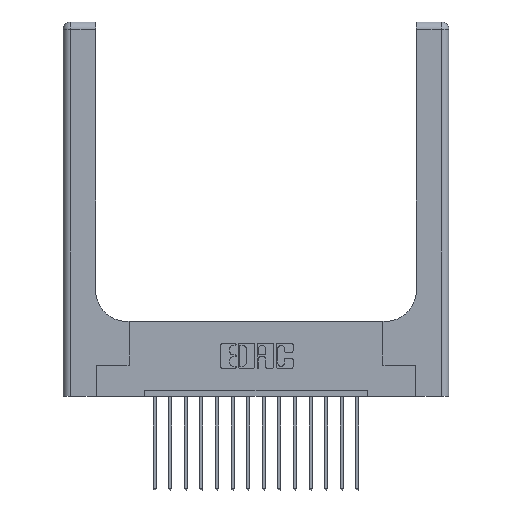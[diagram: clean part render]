
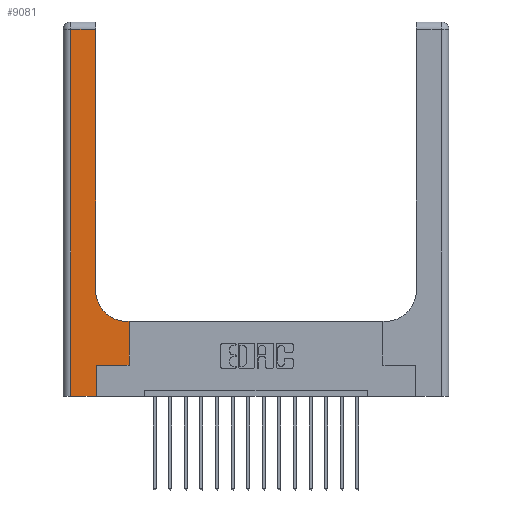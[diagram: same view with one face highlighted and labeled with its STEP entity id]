
A CAD part, top view. The second image highlights one B-rep face of the part: STEP entity #9081.
In plain terms, the highlighted planar face has unit normal (0, 0, 1).
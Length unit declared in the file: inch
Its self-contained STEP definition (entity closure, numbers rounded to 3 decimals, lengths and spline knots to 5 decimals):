
#2 = VECTOR ( 'NONE', #9991, 39.37008 ) ;
#161 = ORIENTED_EDGE ( 'NONE', *, *, #17061, .T. ) ;
#279 = EDGE_LOOP ( 'NONE', ( #14642, #14988, #15880, #3249, #939, #161, #603, #3914, #4945 ) ) ;
#603 = ORIENTED_EDGE ( 'NONE', *, *, #10340, .T. ) ;
#939 = ORIENTED_EDGE ( 'NONE', *, *, #5031, .T. ) ;
#1155 = CARTESIAN_POINT ( 'NONE',  ( 0.528, 0.25, 0.37 ) ) ;
#1302 = DIRECTION ( 'NONE',  ( 0., 1., 0. ) ) ;
#1533 = EDGE_CURVE ( 'NONE', #13329, #9422, #11969, .T. ) ;
#1597 = VECTOR ( 'NONE', #3873, 39.37008 ) ;
#1811 = DIRECTION ( 'NONE',  ( 0., 0., -1. ) ) ;
#2085 = CARTESIAN_POINT ( 'NONE',  ( 0.26, 2.94, 0.37 ) ) ;
#2169 = VECTOR ( 'NONE', #1302, 39.37008 ) ;
#2172 = CARTESIAN_POINT ( 'NONE',  ( 0.06, 2.94, 0.37 ) ) ;
#2354 = VERTEX_POINT ( 'NONE', #2085 ) ;
#2669 = DIRECTION ( 'NONE',  ( 0., 0., -1. ) ) ;
#2956 = LINE ( 'NONE', #17165, #17022 ) ;
#2967 = VERTEX_POINT ( 'NONE', #2172 ) ;
#2977 = CARTESIAN_POINT ( 'NONE',  ( 0., 0., 0.37 ) ) ;
#3102 = VERTEX_POINT ( 'NONE', #13186 ) ;
#3125 = PLANE ( 'NONE',  #13620 ) ;
#3194 = DIRECTION ( 'NONE',  ( 0., -1., 0. ) ) ;
#3249 = ORIENTED_EDGE ( 'NONE', *, *, #1533, .T. ) ;
#3291 = CARTESIAN_POINT ( 'NONE',  ( 0.06, 0., 0.37 ) ) ;
#3873 = DIRECTION ( 'NONE',  ( 0., 1., 0. ) ) ;
#3914 = ORIENTED_EDGE ( 'NONE', *, *, #6206, .T. ) ;
#3915 = CARTESIAN_POINT ( 'NONE',  ( 0.528, 0.25, 0.37 ) ) ;
#4129 = CARTESIAN_POINT ( 'NONE',  ( 0., 2.94, 0.37 ) ) ;
#4898 = DIRECTION ( 'NONE',  ( 1., 0., 0. ) ) ;
#4945 = ORIENTED_EDGE ( 'NONE', *, *, #11742, .T. ) ;
#4989 = VECTOR ( 'NONE', #12416, 39.37008 ) ;
#5031 = EDGE_CURVE ( 'NONE', #9422, #11047, #9626, .T. ) ;
#5335 = VECTOR ( 'NONE', #15311, 39.37008 ) ;
#5460 = FACE_OUTER_BOUND ( 'NONE', #279, .T. ) ;
#5881 = VERTEX_POINT ( 'NONE', #14571 ) ;
#5992 = VECTOR ( 'NONE', #3194, 39.37008 ) ;
#6206 = EDGE_CURVE ( 'NONE', #5881, #3102, #6351, .T. ) ;
#6351 = LINE ( 'NONE', #11103, #2 ) ;
#6656 = DIRECTION ( 'NONE',  ( 1., 0., 0. ) ) ;
#6832 = EDGE_CURVE ( 'NONE', #16754, #2354, #2956, .T. ) ;
#8181 = VERTEX_POINT ( 'NONE', #3915 ) ;
#8361 = LINE ( 'NONE', #16586, #5992 ) ;
#9081 = ADVANCED_FACE ( 'NONE', ( #5460 ), #3125, .F. ) ;
#9422 = VERTEX_POINT ( 'NONE', #13114 ) ;
#9480 = CARTESIAN_POINT ( 'NONE',  ( 0.51, 0.85, 0.37 ) ) ;
#9506 = LINE ( 'NONE', #1155, #1597 ) ;
#9598 = CARTESIAN_POINT ( 'NONE',  ( 0.26, 0.85, 0.37 ) ) ;
#9626 = LINE ( 'NONE', #17626, #2169 ) ;
#9991 = DIRECTION ( 'NONE',  ( -1., 0., 0. ) ) ;
#10340 = EDGE_CURVE ( 'NONE', #8181, #5881, #9506, .T. ) ;
#10349 = DIRECTION ( 'NONE',  ( 0., 1., 0. ) ) ;
#11047 = VERTEX_POINT ( 'NONE', #13972 ) ;
#11103 = CARTESIAN_POINT ( 'NONE',  ( 0.26, 0.6, 0.37 ) ) ;
#11742 = EDGE_CURVE ( 'NONE', #3102, #16754, #14993, .T. ) ;
#11969 = LINE ( 'NONE', #2977, #5335 ) ;
#12053 = EDGE_CURVE ( 'NONE', #2967, #13329, #8361, .T. ) ;
#12416 = DIRECTION ( 'NONE',  ( -1., 0., 0. ) ) ;
#13114 = CARTESIAN_POINT ( 'NONE',  ( 0.265, 0., 0.37 ) ) ;
#13186 = CARTESIAN_POINT ( 'NONE',  ( 0.51, 0.6, 0.37 ) ) ;
#13329 = VERTEX_POINT ( 'NONE', #3291 ) ;
#13620 = AXIS2_PLACEMENT_3D ( 'NONE', #16824, #1811, #16576 ) ;
#13972 = CARTESIAN_POINT ( 'NONE',  ( 0.265, 0.25, 0.37 ) ) ;
#14132 = VECTOR ( 'NONE', #4898, 39.37008 ) ;
#14557 = LINE ( 'NONE', #15698, #14132 ) ;
#14571 = CARTESIAN_POINT ( 'NONE',  ( 0.528, 0.6, 0.37 ) ) ;
#14642 = ORIENTED_EDGE ( 'NONE', *, *, #6832, .T. ) ;
#14988 = ORIENTED_EDGE ( 'NONE', *, *, #15667, .T. ) ;
#14993 = CIRCLE ( 'NONE', #17667, 0.25 ) ;
#15311 = DIRECTION ( 'NONE',  ( 1., 0., 0. ) ) ;
#15667 = EDGE_CURVE ( 'NONE', #2354, #2967, #16730, .T. ) ;
#15698 = CARTESIAN_POINT ( 'NONE',  ( 0.265, 0.25, 0.37 ) ) ;
#15880 = ORIENTED_EDGE ( 'NONE', *, *, #12053, .T. ) ;
#16576 = DIRECTION ( 'NONE',  ( -1., 0., 0. ) ) ;
#16586 = CARTESIAN_POINT ( 'NONE',  ( 0.06, 3., 0.37 ) ) ;
#16730 = LINE ( 'NONE', #4129, #4989 ) ;
#16754 = VERTEX_POINT ( 'NONE', #9598 ) ;
#16824 = CARTESIAN_POINT ( 'NONE',  ( 0., 3., 0.37 ) ) ;
#17022 = VECTOR ( 'NONE', #10349, 39.37008 ) ;
#17061 = EDGE_CURVE ( 'NONE', #11047, #8181, #14557, .T. ) ;
#17165 = CARTESIAN_POINT ( 'NONE',  ( 0.26, 3., 0.37 ) ) ;
#17626 = CARTESIAN_POINT ( 'NONE',  ( 0.265, 0., 0.37 ) ) ;
#17667 = AXIS2_PLACEMENT_3D ( 'NONE', #9480, #2669, #6656 ) ;
